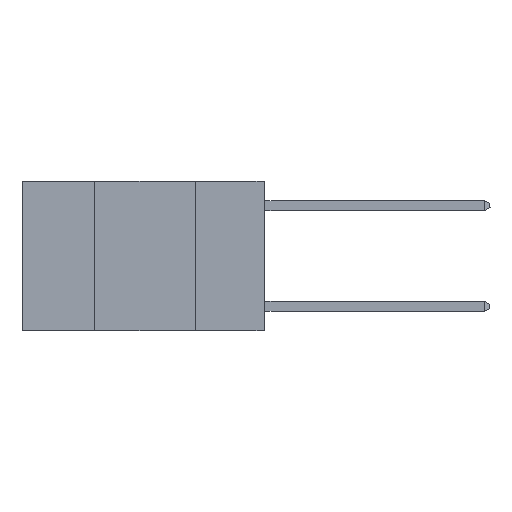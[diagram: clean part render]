
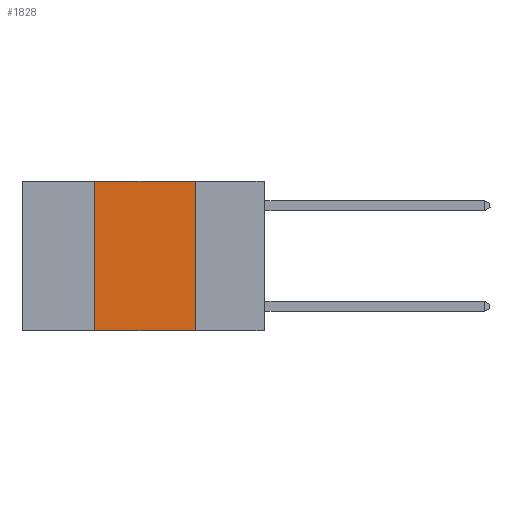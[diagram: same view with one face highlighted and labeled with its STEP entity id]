
A CAD part, left-side view. The second image highlights one B-rep face of the part: STEP entity #1828.
In plain terms, the highlighted planar face has unit normal (-1, 0, 0).
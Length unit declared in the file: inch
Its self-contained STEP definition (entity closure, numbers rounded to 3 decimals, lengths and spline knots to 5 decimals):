
#1 = DIRECTION ( 'NONE',  ( 0., -1., 0. ) ) ;
#795 = DIRECTION ( 'NONE',  ( 0., 0., 1. ) ) ;
#1828 = ADVANCED_FACE ( 'NONE', ( #21552 ), #7996, .F. ) ;
#2084 = VECTOR ( 'NONE', #21650, 39.37008 ) ;
#2925 = CARTESIAN_POINT ( 'NONE',  ( 0., 0.6, 0. ) ) ;
#4642 = DIRECTION ( 'NONE',  ( 0., 0., -1. ) ) ;
#4805 = ORIENTED_EDGE ( 'NONE', *, *, #14974, .F. ) ;
#5200 = DIRECTION ( 'NONE',  ( 0., -1., 0. ) ) ;
#5322 = ORIENTED_EDGE ( 'NONE', *, *, #20965, .T. ) ;
#5662 = VERTEX_POINT ( 'NONE', #17902 ) ;
#7502 = VECTOR ( 'NONE', #795, 39.37008 ) ;
#7651 = CARTESIAN_POINT ( 'NONE',  ( 0., 0.42, 0. ) ) ;
#7996 = PLANE ( 'NONE',  #16986 ) ;
#8098 = VECTOR ( 'NONE', #1, 39.37008 ) ;
#10068 = CARTESIAN_POINT ( 'NONE',  ( 0., 0.42, 0. ) ) ;
#10201 = CARTESIAN_POINT ( 'NONE',  ( 0., 0.6, 0. ) ) ;
#10262 = CARTESIAN_POINT ( 'NONE',  ( 0., 0.6, -0.37 ) ) ;
#10483 = VERTEX_POINT ( 'NONE', #10068 ) ;
#11496 = CARTESIAN_POINT ( 'NONE',  ( 0., 0.17, 0. ) ) ;
#11594 = EDGE_CURVE ( 'NONE', #5662, #10483, #15941, .T. ) ;
#12580 = LINE ( 'NONE', #10201, #8098 ) ;
#13802 = ORIENTED_EDGE ( 'NONE', *, *, #18494, .F. ) ;
#14764 = EDGE_LOOP ( 'NONE', ( #4805, #13802, #18260, #5322 ) ) ;
#14782 = DIRECTION ( 'NONE',  ( 1., 0., 0. ) ) ;
#14974 = EDGE_CURVE ( 'NONE', #21510, #18462, #20073, .T. ) ;
#15505 = VECTOR ( 'NONE', #5200, 39.37008 ) ;
#15941 = LINE ( 'NONE', #7651, #7502 ) ;
#16053 = LINE ( 'NONE', #10262, #15505 ) ;
#16631 = CARTESIAN_POINT ( 'NONE',  ( 0., 0.17, 0. ) ) ;
#16986 = AXIS2_PLACEMENT_3D ( 'NONE', #2925, #14782, #4642 ) ;
#17902 = CARTESIAN_POINT ( 'NONE',  ( 0., 0.42, -0.37 ) ) ;
#18260 = ORIENTED_EDGE ( 'NONE', *, *, #11594, .F. ) ;
#18462 = VERTEX_POINT ( 'NONE', #21806 ) ;
#18494 = EDGE_CURVE ( 'NONE', #10483, #21510, #12580, .T. ) ;
#20073 = LINE ( 'NONE', #16631, #2084 ) ;
#20965 = EDGE_CURVE ( 'NONE', #5662, #18462, #16053, .T. ) ;
#21510 = VERTEX_POINT ( 'NONE', #11496 ) ;
#21552 = FACE_OUTER_BOUND ( 'NONE', #14764, .T. ) ;
#21650 = DIRECTION ( 'NONE',  ( 0., 0., -1. ) ) ;
#21806 = CARTESIAN_POINT ( 'NONE',  ( 0., 0.17, -0.37 ) ) ;
